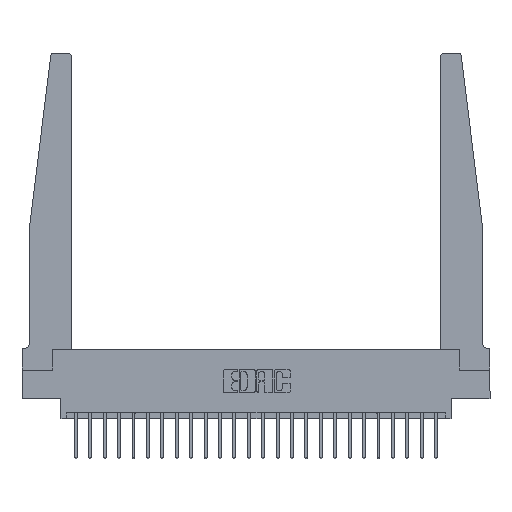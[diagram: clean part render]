
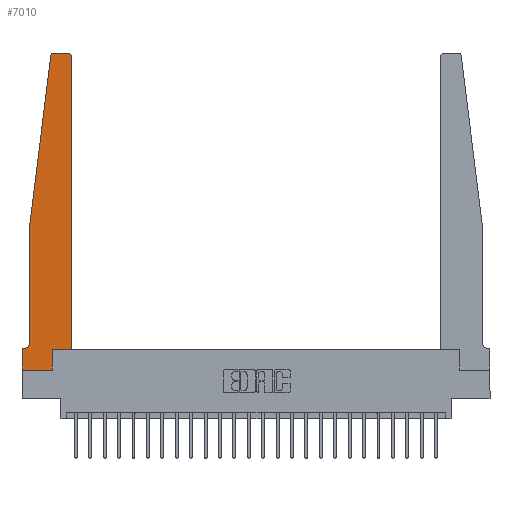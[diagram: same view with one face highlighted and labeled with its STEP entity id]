
A CAD part, top view. The second image highlights one B-rep face of the part: STEP entity #7010.
In plain terms, the highlighted planar face has unit normal (0, 0, 1).
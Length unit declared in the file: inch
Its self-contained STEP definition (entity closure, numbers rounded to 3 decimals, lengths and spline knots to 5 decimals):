
#58 = PLANE ( 'NONE',  #17273 ) ;
#522 = VECTOR ( 'NONE', #8280, 39.37008 ) ;
#796 = EDGE_LOOP ( 'NONE', ( #7916, #22705, #4662, #6890, #7427, #18493, #5170, #9882, #1497, #16651, #11612, #12540 ) ) ;
#1115 = EDGE_CURVE ( 'NONE', #18378, #20498, #7508, .T. ) ;
#1497 = ORIENTED_EDGE ( 'NONE', *, *, #18277, .T. ) ;
#1918 = LINE ( 'NONE', #9317, #16230 ) ;
#2369 = VECTOR ( 'NONE', #2389, 39.37008 ) ;
#2389 = DIRECTION ( 'NONE',  ( 1., 0., 0. ) ) ;
#2675 = CARTESIAN_POINT ( 'NONE',  ( 0., 0.1875, 0.37 ) ) ;
#3044 = DIRECTION ( 'NONE',  ( 0., 0., -1. ) ) ;
#3080 = LINE ( 'NONE', #22121, #16808 ) ;
#3361 = VERTEX_POINT ( 'NONE', #13474 ) ;
#3581 = DIRECTION ( 'NONE',  ( -0.122, -0.992, 0. ) ) ;
#4468 = CARTESIAN_POINT ( 'NONE',  ( 0.395, 2.72, 0.37 ) ) ;
#4556 = VECTOR ( 'NONE', #18966, 39.37008 ) ;
#4662 = ORIENTED_EDGE ( 'NONE', *, *, #6924, .T. ) ;
#5170 = ORIENTED_EDGE ( 'NONE', *, *, #6967, .T. ) ;
#5516 = LINE ( 'NONE', #6422, #522 ) ;
#5592 = VERTEX_POINT ( 'NONE', #13913 ) ;
#5696 = DIRECTION ( 'NONE',  ( 0., 0., 1. ) ) ;
#5834 = CIRCLE ( 'NONE', #10794, 0.03 ) ;
#6335 = DIRECTION ( 'NONE',  ( 1., 0., 0. ) ) ;
#6422 = CARTESIAN_POINT ( 'NONE',  ( 0.065, 1.25, 0.37 ) ) ;
#6697 = DIRECTION ( 'NONE',  ( 0., 1., 0. ) ) ;
#6723 = CARTESIAN_POINT ( 'NONE',  ( 0.2605, 0.18, 0.37 ) ) ;
#6890 = ORIENTED_EDGE ( 'NONE', *, *, #11995, .T. ) ;
#6924 = EDGE_CURVE ( 'NONE', #21168, #16168, #3080, .T. ) ;
#6967 = EDGE_CURVE ( 'NONE', #20498, #5592, #1918, .T. ) ;
#7010 = ADVANCED_FACE ( 'NONE', ( #19400 ), #58, .T. ) ;
#7100 = EDGE_CURVE ( 'NONE', #13235, #3361, #8326, .T. ) ;
#7104 = VECTOR ( 'NONE', #8595, 39.37008 ) ;
#7188 = AXIS2_PLACEMENT_3D ( 'NONE', #14251, #3044, #16109 ) ;
#7364 = CARTESIAN_POINT ( 'NONE',  ( 0., 0., 0.37 ) ) ;
#7427 = ORIENTED_EDGE ( 'NONE', *, *, #10214, .T. ) ;
#7508 = LINE ( 'NONE', #16266, #15681 ) ;
#7880 = CIRCLE ( 'NONE', #7188, 0.05 ) ;
#7916 = ORIENTED_EDGE ( 'NONE', *, *, #7100, .T. ) ;
#7952 = LINE ( 'NONE', #7364, #22771 ) ;
#8070 = VERTEX_POINT ( 'NONE', #10805 ) ;
#8138 = CIRCLE ( 'NONE', #20008, 0.03 ) ;
#8222 = DIRECTION ( 'NONE',  ( 0., 0., 1. ) ) ;
#8280 = DIRECTION ( 'NONE',  ( 0., -1., 0. ) ) ;
#8326 = LINE ( 'NONE', #15245, #4556 ) ;
#8595 = DIRECTION ( 'NONE',  ( 0., 1., 0. ) ) ;
#8775 = DIRECTION ( 'NONE',  ( -1., 0., 0. ) ) ;
#9206 = CARTESIAN_POINT ( 'NONE',  ( 0.065, 1.25, 0.37 ) ) ;
#9276 = VECTOR ( 'NONE', #6697, 39.37008 ) ;
#9317 = CARTESIAN_POINT ( 'NONE',  ( 0., 0., 0.37 ) ) ;
#9882 = ORIENTED_EDGE ( 'NONE', *, *, #20165, .T. ) ;
#10214 = EDGE_CURVE ( 'NONE', #11161, #18378, #7880, .T. ) ;
#10507 = EDGE_CURVE ( 'NONE', #22286, #19546, #12910, .T. ) ;
#10794 = AXIS2_PLACEMENT_3D ( 'NONE', #19376, #8222, #21234 ) ;
#10805 = CARTESIAN_POINT ( 'NONE',  ( 0.425, 2.72, 0.37 ) ) ;
#11161 = VERTEX_POINT ( 'NONE', #22675 ) ;
#11249 = EDGE_CURVE ( 'NONE', #3361, #21168, #5834, .T. ) ;
#11612 = ORIENTED_EDGE ( 'NONE', *, *, #15278, .T. ) ;
#11700 = CARTESIAN_POINT ( 'NONE',  ( 0.425, 0.18, 0.37 ) ) ;
#11995 = EDGE_CURVE ( 'NONE', #16168, #11161, #5516, .T. ) ;
#12540 = ORIENTED_EDGE ( 'NONE', *, *, #14000, .T. ) ;
#12910 = LINE ( 'NONE', #11700, #2369 ) ;
#13235 = VERTEX_POINT ( 'NONE', #13301 ) ;
#13301 = CARTESIAN_POINT ( 'NONE',  ( 0.395, 2.75, 0.37 ) ) ;
#13433 = VERTEX_POINT ( 'NONE', #23074 ) ;
#13474 = CARTESIAN_POINT ( 'NONE',  ( 0.27653, 2.75, 0.37 ) ) ;
#13860 = CARTESIAN_POINT ( 'NONE',  ( 0.2605, 0.18, 0.37 ) ) ;
#13913 = CARTESIAN_POINT ( 'NONE',  ( 0., 0., 0.37 ) ) ;
#14000 = EDGE_CURVE ( 'NONE', #8070, #13235, #8138, .T. ) ;
#14251 = CARTESIAN_POINT ( 'NONE',  ( 0.015, 0.2375, 0.37 ) ) ;
#14474 = CARTESIAN_POINT ( 'NONE',  ( 0.015, 0.1875, 0.37 ) ) ;
#14860 = DIRECTION ( 'NONE',  ( 0., -1., 0. ) ) ;
#15245 = CARTESIAN_POINT ( 'NONE',  ( 0.25, 2.75, 0.37 ) ) ;
#15278 = EDGE_CURVE ( 'NONE', #19546, #8070, #19144, .T. ) ;
#15681 = VECTOR ( 'NONE', #8775, 39.37008 ) ;
#16109 = DIRECTION ( 'NONE',  ( -1., 0., 0. ) ) ;
#16168 = VERTEX_POINT ( 'NONE', #9206 ) ;
#16230 = VECTOR ( 'NONE', #14860, 39.37008 ) ;
#16266 = CARTESIAN_POINT ( 'NONE',  ( 0.065, 0.1875, 0.37 ) ) ;
#16651 = ORIENTED_EDGE ( 'NONE', *, *, #10507, .T. ) ;
#16808 = VECTOR ( 'NONE', #3581, 39.37008 ) ;
#16868 = CARTESIAN_POINT ( 'NONE',  ( 0., 0.1875, 0.37 ) ) ;
#17011 = LINE ( 'NONE', #6723, #7104 ) ;
#17273 = AXIS2_PLACEMENT_3D ( 'NONE', #16868, #5696, #18737 ) ;
#17494 = DIRECTION ( 'NONE',  ( 0., 0., 1. ) ) ;
#18277 = EDGE_CURVE ( 'NONE', #13433, #22286, #17011, .T. ) ;
#18378 = VERTEX_POINT ( 'NONE', #14474 ) ;
#18493 = ORIENTED_EDGE ( 'NONE', *, *, #1115, .T. ) ;
#18737 = DIRECTION ( 'NONE',  ( 1., 0., 0. ) ) ;
#18966 = DIRECTION ( 'NONE',  ( -1., 0., 0. ) ) ;
#19144 = LINE ( 'NONE', #19619, #9276 ) ;
#19376 = CARTESIAN_POINT ( 'NONE',  ( 0.27653, 2.72, 0.37 ) ) ;
#19400 = FACE_OUTER_BOUND ( 'NONE', #796, .T. ) ;
#19546 = VERTEX_POINT ( 'NONE', #19838 ) ;
#19619 = CARTESIAN_POINT ( 'NONE',  ( 0.425, 0.18, 0.37 ) ) ;
#19838 = CARTESIAN_POINT ( 'NONE',  ( 0.425, 0.18, 0.37 ) ) ;
#20008 = AXIS2_PLACEMENT_3D ( 'NONE', #4468, #17494, #6335 ) ;
#20165 = EDGE_CURVE ( 'NONE', #5592, #13433, #7952, .T. ) ;
#20373 = DIRECTION ( 'NONE',  ( 1., 0., 0. ) ) ;
#20498 = VERTEX_POINT ( 'NONE', #2675 ) ;
#21168 = VERTEX_POINT ( 'NONE', #21267 ) ;
#21234 = DIRECTION ( 'NONE',  ( 1., 0., 0. ) ) ;
#21267 = CARTESIAN_POINT ( 'NONE',  ( 0.24675, 2.72367, 0.37 ) ) ;
#22121 = CARTESIAN_POINT ( 'NONE',  ( 0.065, 1.25, 0.37 ) ) ;
#22286 = VERTEX_POINT ( 'NONE', #13860 ) ;
#22675 = CARTESIAN_POINT ( 'NONE',  ( 0.065, 0.2375, 0.37 ) ) ;
#22705 = ORIENTED_EDGE ( 'NONE', *, *, #11249, .T. ) ;
#22771 = VECTOR ( 'NONE', #20373, 39.37008 ) ;
#23074 = CARTESIAN_POINT ( 'NONE',  ( 0.2605, 0., 0.37 ) ) ;
